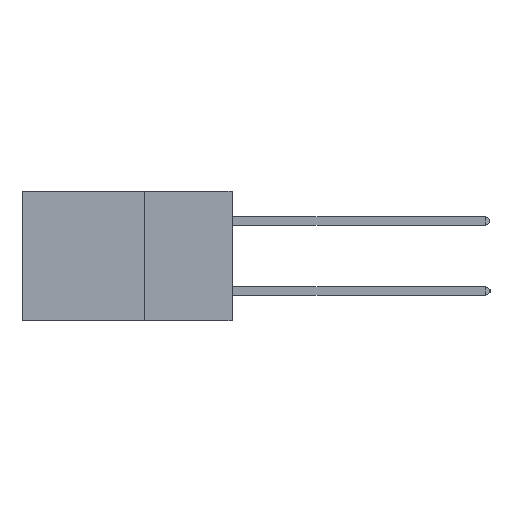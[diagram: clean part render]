
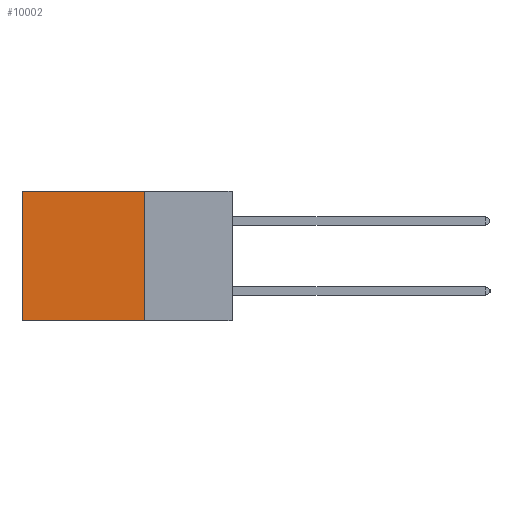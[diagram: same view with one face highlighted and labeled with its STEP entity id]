
A CAD part, left-side view. The second image highlights one B-rep face of the part: STEP entity #10002.
In plain terms, the highlighted planar face has unit normal (-1, 0, 0).
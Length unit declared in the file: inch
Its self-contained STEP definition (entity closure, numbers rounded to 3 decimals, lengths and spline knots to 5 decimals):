
#299 = CARTESIAN_POINT ( 'NONE',  ( 0.2875, 0.25, 0. ) ) ;
#355 = LINE ( 'NONE', #17106, #12626 ) ;
#934 = CARTESIAN_POINT ( 'NONE',  ( 0.2875, 0.25, -0.37 ) ) ;
#2076 = CARTESIAN_POINT ( 'NONE',  ( 0.2875, 0.25, -0.37 ) ) ;
#2381 = ORIENTED_EDGE ( 'NONE', *, *, #13438, .F. ) ;
#3703 = DIRECTION ( 'NONE',  ( 0., 1., 0. ) ) ;
#4013 = VECTOR ( 'NONE', #18796, 39.37008 ) ;
#5967 = DIRECTION ( 'NONE',  ( 0., 0., -1. ) ) ;
#6266 = AXIS2_PLACEMENT_3D ( 'NONE', #299, #19463, #9955 ) ;
#7000 = EDGE_CURVE ( 'NONE', #14228, #13407, #18101, .T. ) ;
#7097 = DIRECTION ( 'NONE',  ( 0., 0., -1. ) ) ;
#7675 = LINE ( 'NONE', #7710, #4013 ) ;
#7710 = CARTESIAN_POINT ( 'NONE',  ( 0.2875, 0.25, 0. ) ) ;
#7859 = VECTOR ( 'NONE', #7097, 39.37008 ) ;
#8329 = PLANE ( 'NONE',  #6266 ) ;
#9643 = VECTOR ( 'NONE', #3703, 39.37008 ) ;
#9955 = DIRECTION ( 'NONE',  ( 0., 0., -1. ) ) ;
#10002 = ADVANCED_FACE ( 'NONE', ( #13046 ), #8329, .F. ) ;
#11062 = CARTESIAN_POINT ( 'NONE',  ( 0.2875, 0.25, 0. ) ) ;
#11833 = EDGE_CURVE ( 'NONE', #12459, #17419, #7675, .T. ) ;
#12322 = CARTESIAN_POINT ( 'NONE',  ( 0.2875, 0.6, 0. ) ) ;
#12459 = VERTEX_POINT ( 'NONE', #11062 ) ;
#12626 = VECTOR ( 'NONE', #5967, 39.37008 ) ;
#13046 = FACE_OUTER_BOUND ( 'NONE', #16480, .T. ) ;
#13407 = VERTEX_POINT ( 'NONE', #13413 ) ;
#13413 = CARTESIAN_POINT ( 'NONE',  ( 0.2875, 0.6, -0.37 ) ) ;
#13438 = EDGE_CURVE ( 'NONE', #12459, #14228, #19555, .T. ) ;
#14228 = VERTEX_POINT ( 'NONE', #934 ) ;
#14855 = EDGE_CURVE ( 'NONE', #17419, #13407, #355, .T. ) ;
#16480 = EDGE_LOOP ( 'NONE', ( #16523, #18660, #2381, #19443 ) ) ;
#16523 = ORIENTED_EDGE ( 'NONE', *, *, #14855, .T. ) ;
#16672 = CARTESIAN_POINT ( 'NONE',  ( 0.2875, 0.25, 0. ) ) ;
#17106 = CARTESIAN_POINT ( 'NONE',  ( 0.2875, 0.6, 0. ) ) ;
#17419 = VERTEX_POINT ( 'NONE', #12322 ) ;
#18101 = LINE ( 'NONE', #2076, #9643 ) ;
#18660 = ORIENTED_EDGE ( 'NONE', *, *, #7000, .F. ) ;
#18796 = DIRECTION ( 'NONE',  ( 0., 1., 0. ) ) ;
#19443 = ORIENTED_EDGE ( 'NONE', *, *, #11833, .T. ) ;
#19463 = DIRECTION ( 'NONE',  ( 1., 0., 0. ) ) ;
#19555 = LINE ( 'NONE', #16672, #7859 ) ;
